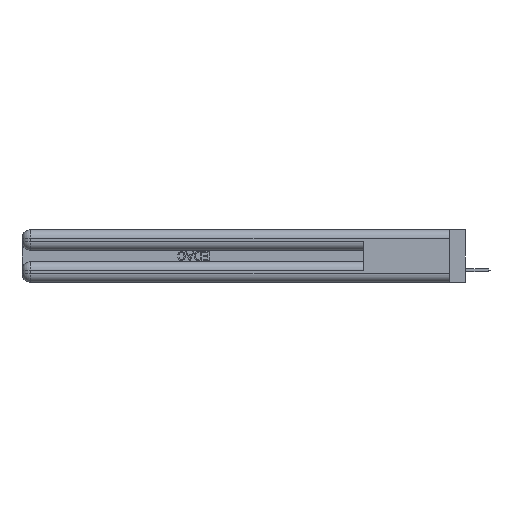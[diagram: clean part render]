
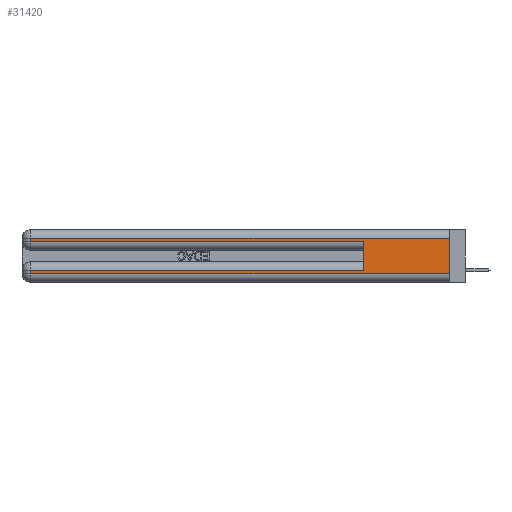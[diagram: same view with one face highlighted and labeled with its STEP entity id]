
A CAD part, left-side view. The second image highlights one B-rep face of the part: STEP entity #31420.
In plain terms, the highlighted planar face has unit normal (-1, 0, 0).
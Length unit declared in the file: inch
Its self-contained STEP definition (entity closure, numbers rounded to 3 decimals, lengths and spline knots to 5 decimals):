
#1570 = LINE ( 'NONE', #31118, #18692 ) ;
#1699 = DIRECTION ( 'NONE',  ( 0., 1., 0. ) ) ;
#3174 = CARTESIAN_POINT ( 'NONE',  ( 0., 0., 0.31 ) ) ;
#5224 = EDGE_CURVE ( 'NONE', #33619, #38815, #50207, .T. ) ;
#5369 = CARTESIAN_POINT ( 'NONE',  ( 0., 2.94, 0.37 ) ) ;
#5594 = ORIENTED_EDGE ( 'NONE', *, *, #30356, .T. ) ;
#7162 = CARTESIAN_POINT ( 'NONE',  ( 0., 0., 0.06 ) ) ;
#7379 = ORIENTED_EDGE ( 'NONE', *, *, #15286, .F. ) ;
#9707 = CARTESIAN_POINT ( 'NONE',  ( 0., 0.6, 0.085 ) ) ;
#10190 = AXIS2_PLACEMENT_3D ( 'NONE', #28939, #49450, #24309 ) ;
#10510 = VECTOR ( 'NONE', #13131, 39.37008 ) ;
#10549 = VERTEX_POINT ( 'NONE', #23904 ) ;
#10575 = CARTESIAN_POINT ( 'NONE',  ( 0., 2.94, 0.085 ) ) ;
#12117 = EDGE_CURVE ( 'NONE', #37798, #27194, #52248, .T. ) ;
#13131 = DIRECTION ( 'NONE',  ( 0., 0., 1. ) ) ;
#13222 = ORIENTED_EDGE ( 'NONE', *, *, #30203, .T. ) ;
#14155 = CARTESIAN_POINT ( 'NONE',  ( 0., 2.94, 0.31 ) ) ;
#15286 = EDGE_CURVE ( 'NONE', #53367, #51312, #25172, .T. ) ;
#16476 = VERTEX_POINT ( 'NONE', #36368 ) ;
#16811 = ORIENTED_EDGE ( 'NONE', *, *, #5224, .T. ) ;
#17485 = VECTOR ( 'NONE', #1699, 39.37008 ) ;
#17510 = DIRECTION ( 'NONE',  ( 0., 1., 0. ) ) ;
#18075 = CARTESIAN_POINT ( 'NONE',  ( 0., 0., 0.085 ) ) ;
#18229 = DIRECTION ( 'NONE',  ( 0., 0., -1. ) ) ;
#18520 = CARTESIAN_POINT ( 'NONE',  ( 0., 0., 0.31 ) ) ;
#18547 = EDGE_CURVE ( 'NONE', #16476, #51312, #23919, .T. ) ;
#18692 = VECTOR ( 'NONE', #39540, 39.37008 ) ;
#22582 = CARTESIAN_POINT ( 'NONE',  ( 0., 2.94, 0.285 ) ) ;
#22619 = VECTOR ( 'NONE', #17510, 39.37008 ) ;
#23383 = DIRECTION ( 'NONE',  ( 0., 0., -1. ) ) ;
#23742 = PLANE ( 'NONE',  #10190 ) ;
#23904 = CARTESIAN_POINT ( 'NONE',  ( 0., 0.6, 0.285 ) ) ;
#23919 = LINE ( 'NONE', #51149, #25249 ) ;
#24309 = DIRECTION ( 'NONE',  ( 0., 0., -1. ) ) ;
#24802 = EDGE_CURVE ( 'NONE', #37798, #10549, #32951, .T. ) ;
#25172 = LINE ( 'NONE', #48503, #49445 ) ;
#25249 = VECTOR ( 'NONE', #51316, 39.37008 ) ;
#27194 = VERTEX_POINT ( 'NONE', #10575 ) ;
#28317 = ORIENTED_EDGE ( 'NONE', *, *, #43195, .T. ) ;
#28939 = CARTESIAN_POINT ( 'NONE',  ( 0., 0., 0.37 ) ) ;
#30203 = EDGE_CURVE ( 'NONE', #38815, #10549, #1570, .T. ) ;
#30356 = EDGE_CURVE ( 'NONE', #53367, #33619, #49674, .T. ) ;
#30373 = FACE_OUTER_BOUND ( 'NONE', #47396, .T. ) ;
#30810 = LINE ( 'NONE', #5369, #45994 ) ;
#31118 = CARTESIAN_POINT ( 'NONE',  ( 0., 0., 0.285 ) ) ;
#31420 = ADVANCED_FACE ( 'NONE', ( #30373 ), #23742, .F. ) ;
#32210 = ORIENTED_EDGE ( 'NONE', *, *, #24802, .F. ) ;
#32951 = LINE ( 'NONE', #51024, #10510 ) ;
#33619 = VERTEX_POINT ( 'NONE', #14155 ) ;
#36368 = CARTESIAN_POINT ( 'NONE',  ( 0., 2.94, 0.06 ) ) ;
#37798 = VERTEX_POINT ( 'NONE', #9707 ) ;
#38815 = VERTEX_POINT ( 'NONE', #22582 ) ;
#39540 = DIRECTION ( 'NONE',  ( 0., -1., 0. ) ) ;
#40376 = CARTESIAN_POINT ( 'NONE',  ( 0., 2.94, 0.37 ) ) ;
#42966 = ORIENTED_EDGE ( 'NONE', *, *, #18547, .T. ) ;
#43195 = EDGE_CURVE ( 'NONE', #27194, #16476, #30810, .T. ) ;
#45994 = VECTOR ( 'NONE', #50756, 39.37008 ) ;
#46101 = ORIENTED_EDGE ( 'NONE', *, *, #12117, .T. ) ;
#47396 = EDGE_LOOP ( 'NONE', ( #7379, #5594, #16811, #13222, #32210, #46101, #28317, #42966 ) ) ;
#48503 = CARTESIAN_POINT ( 'NONE',  ( 0., 0., 0.37 ) ) ;
#49445 = VECTOR ( 'NONE', #23383, 39.37008 ) ;
#49450 = DIRECTION ( 'NONE',  ( 1., 0., 0. ) ) ;
#49674 = LINE ( 'NONE', #18520, #22619 ) ;
#50207 = LINE ( 'NONE', #40376, #54135 ) ;
#50756 = DIRECTION ( 'NONE',  ( 0., 0., -1. ) ) ;
#51024 = CARTESIAN_POINT ( 'NONE',  ( 0., 0.6, 0.145 ) ) ;
#51149 = CARTESIAN_POINT ( 'NONE',  ( 0., 0., 0.06 ) ) ;
#51312 = VERTEX_POINT ( 'NONE', #7162 ) ;
#51316 = DIRECTION ( 'NONE',  ( 0., -1., 0. ) ) ;
#52248 = LINE ( 'NONE', #18075, #17485 ) ;
#53367 = VERTEX_POINT ( 'NONE', #3174 ) ;
#54135 = VECTOR ( 'NONE', #18229, 39.37008 ) ;
